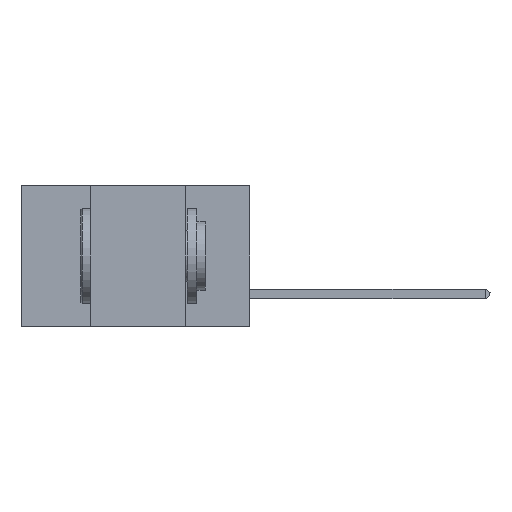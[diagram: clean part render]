
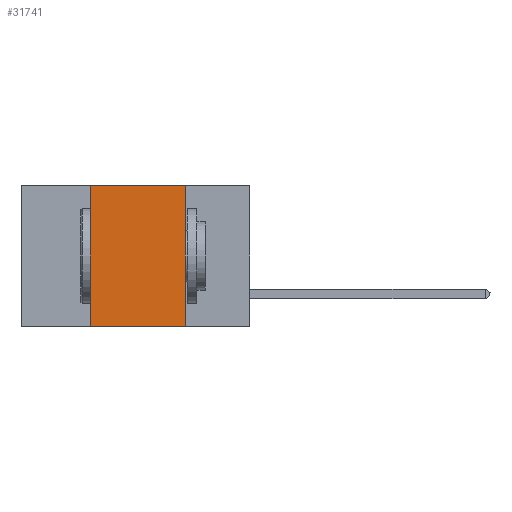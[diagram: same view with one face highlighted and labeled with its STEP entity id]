
A CAD part, left-side view. The second image highlights one B-rep face of the part: STEP entity #31741.
In plain terms, the highlighted planar face has unit normal (-1, 0, 0).
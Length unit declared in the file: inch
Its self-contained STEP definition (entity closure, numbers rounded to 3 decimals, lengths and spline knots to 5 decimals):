
#129 = VECTOR ( 'NONE', #12259, 39.37008 ) ;
#1968 = LINE ( 'NONE', #33151, #4708 ) ;
#4708 = VECTOR ( 'NONE', #19086, 39.37008 ) ;
#4832 = ORIENTED_EDGE ( 'NONE', *, *, #15250, .F. ) ;
#7864 = CARTESIAN_POINT ( 'NONE',  ( 0., 0.17, -0.37 ) ) ;
#9194 = VERTEX_POINT ( 'NONE', #32524 ) ;
#11247 = ORIENTED_EDGE ( 'NONE', *, *, #18650, .T. ) ;
#12259 = DIRECTION ( 'NONE',  ( 0., 0., 1. ) ) ;
#13112 = DIRECTION ( 'NONE',  ( 0., 0., -1. ) ) ;
#13499 = CARTESIAN_POINT ( 'NONE',  ( 0., 0.6, -0.37 ) ) ;
#13792 = CARTESIAN_POINT ( 'NONE',  ( 0., 0.17, 0. ) ) ;
#14633 = EDGE_CURVE ( 'NONE', #9194, #33663, #1968, .T. ) ;
#14798 = VERTEX_POINT ( 'NONE', #23872 ) ;
#15250 = EDGE_CURVE ( 'NONE', #33663, #35020, #25354, .T. ) ;
#15444 = CARTESIAN_POINT ( 'NONE',  ( 0., 0.42, 0. ) ) ;
#16579 = LINE ( 'NONE', #13499, #34625 ) ;
#16975 = DIRECTION ( 'NONE',  ( 0., 0., -1. ) ) ;
#18650 = EDGE_CURVE ( 'NONE', #14798, #35020, #16579, .T. ) ;
#19086 = DIRECTION ( 'NONE',  ( 0., -1., 0. ) ) ;
#19175 = ORIENTED_EDGE ( 'NONE', *, *, #32697, .F. ) ;
#20004 = CARTESIAN_POINT ( 'NONE',  ( 0., 0.6, 0. ) ) ;
#22882 = EDGE_LOOP ( 'NONE', ( #4832, #27030, #19175, #11247 ) ) ;
#23872 = CARTESIAN_POINT ( 'NONE',  ( 0., 0.42, -0.37 ) ) ;
#24591 = AXIS2_PLACEMENT_3D ( 'NONE', #20004, #34135, #16975 ) ;
#25354 = LINE ( 'NONE', #30496, #34808 ) ;
#25402 = PLANE ( 'NONE',  #24591 ) ;
#25417 = FACE_OUTER_BOUND ( 'NONE', #22882, .T. ) ;
#26205 = LINE ( 'NONE', #15444, #129 ) ;
#27030 = ORIENTED_EDGE ( 'NONE', *, *, #14633, .F. ) ;
#30496 = CARTESIAN_POINT ( 'NONE',  ( 0., 0.17, 0. ) ) ;
#31741 = ADVANCED_FACE ( 'NONE', ( #25417 ), #25402, .F. ) ;
#32524 = CARTESIAN_POINT ( 'NONE',  ( 0., 0.42, 0. ) ) ;
#32697 = EDGE_CURVE ( 'NONE', #14798, #9194, #26205, .T. ) ;
#33076 = DIRECTION ( 'NONE',  ( 0., -1., 0. ) ) ;
#33151 = CARTESIAN_POINT ( 'NONE',  ( 0., 0.6, 0. ) ) ;
#33663 = VERTEX_POINT ( 'NONE', #13792 ) ;
#34135 = DIRECTION ( 'NONE',  ( 1., 0., 0. ) ) ;
#34625 = VECTOR ( 'NONE', #33076, 39.37008 ) ;
#34808 = VECTOR ( 'NONE', #13112, 39.37008 ) ;
#35020 = VERTEX_POINT ( 'NONE', #7864 ) ;
